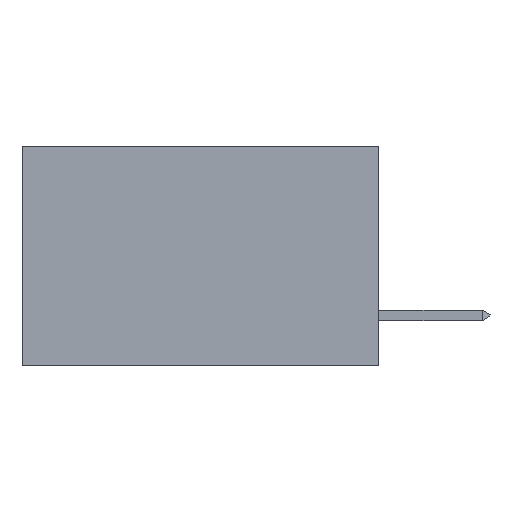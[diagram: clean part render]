
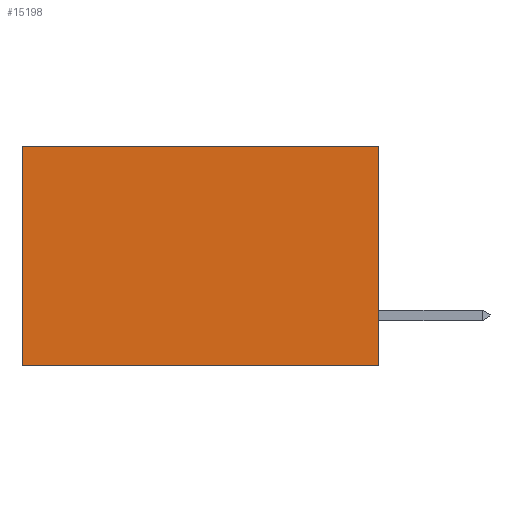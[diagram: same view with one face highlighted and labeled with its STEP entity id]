
A CAD part, left-side view. The second image highlights one B-rep face of the part: STEP entity #15198.
In plain terms, the highlighted planar face has unit normal (-1, 0, 0).
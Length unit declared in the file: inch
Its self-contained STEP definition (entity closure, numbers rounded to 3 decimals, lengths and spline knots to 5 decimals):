
#504 = DIRECTION ( 'NONE',  ( 0., 0., -1. ) ) ;
#744 = DIRECTION ( 'NONE',  ( 1., 0., 0. ) ) ;
#2187 = LINE ( 'NONE', #20095, #19344 ) ;
#3140 = LINE ( 'NONE', #11646, #6062 ) ;
#4602 = EDGE_LOOP ( 'NONE', ( #10928, #8521, #21330, #19048 ) ) ;
#5298 = DIRECTION ( 'NONE',  ( 0., 0., -1. ) ) ;
#5418 = VECTOR ( 'NONE', #5298, 39.37008 ) ;
#6062 = VECTOR ( 'NONE', #6665, 39.37008 ) ;
#6385 = CARTESIAN_POINT ( 'NONE',  ( 0.2615, 0., -0.37 ) ) ;
#6605 = CARTESIAN_POINT ( 'NONE',  ( 0.2615, 0., -0.37 ) ) ;
#6665 = DIRECTION ( 'NONE',  ( 0., 1., 0. ) ) ;
#7007 = VERTEX_POINT ( 'NONE', #8806 ) ;
#7392 = CARTESIAN_POINT ( 'NONE',  ( 0.2615, 0., -0.37 ) ) ;
#7435 = VERTEX_POINT ( 'NONE', #20485 ) ;
#8115 = CARTESIAN_POINT ( 'NONE',  ( 0.2615, 0.6, -0.37 ) ) ;
#8517 = EDGE_CURVE ( 'NONE', #7007, #20337, #17441, .T. ) ;
#8521 = ORIENTED_EDGE ( 'NONE', *, *, #12349, .F. ) ;
#8806 = CARTESIAN_POINT ( 'NONE',  ( 0.2615, 0.6, 0. ) ) ;
#10381 = AXIS2_PLACEMENT_3D ( 'NONE', #6385, #744, #504 ) ;
#10928 = ORIENTED_EDGE ( 'NONE', *, *, #8517, .T. ) ;
#11226 = PLANE ( 'NONE',  #10381 ) ;
#11646 = CARTESIAN_POINT ( 'NONE',  ( 0.2615, 0., 0. ) ) ;
#12349 = EDGE_CURVE ( 'NONE', #13355, #20337, #2187, .T. ) ;
#13355 = VERTEX_POINT ( 'NONE', #7392 ) ;
#14853 = LINE ( 'NONE', #6605, #19129 ) ;
#15198 = ADVANCED_FACE ( 'NONE', ( #16731 ), #11226, .F. ) ;
#15803 = CARTESIAN_POINT ( 'NONE',  ( 0.2615, 0.6, -0.37 ) ) ;
#16731 = FACE_OUTER_BOUND ( 'NONE', #4602, .T. ) ;
#17441 = LINE ( 'NONE', #15803, #5418 ) ;
#18417 = EDGE_CURVE ( 'NONE', #7435, #13355, #14853, .T. ) ;
#18670 = EDGE_CURVE ( 'NONE', #7435, #7007, #3140, .T. ) ;
#19048 = ORIENTED_EDGE ( 'NONE', *, *, #18670, .T. ) ;
#19129 = VECTOR ( 'NONE', #21939, 39.37008 ) ;
#19344 = VECTOR ( 'NONE', #21860, 39.37008 ) ;
#20095 = CARTESIAN_POINT ( 'NONE',  ( 0.2615, 0., -0.37 ) ) ;
#20337 = VERTEX_POINT ( 'NONE', #8115 ) ;
#20485 = CARTESIAN_POINT ( 'NONE',  ( 0.2615, 0., 0. ) ) ;
#21330 = ORIENTED_EDGE ( 'NONE', *, *, #18417, .F. ) ;
#21860 = DIRECTION ( 'NONE',  ( 0., 1., 0. ) ) ;
#21939 = DIRECTION ( 'NONE',  ( 0., 0., -1. ) ) ;
